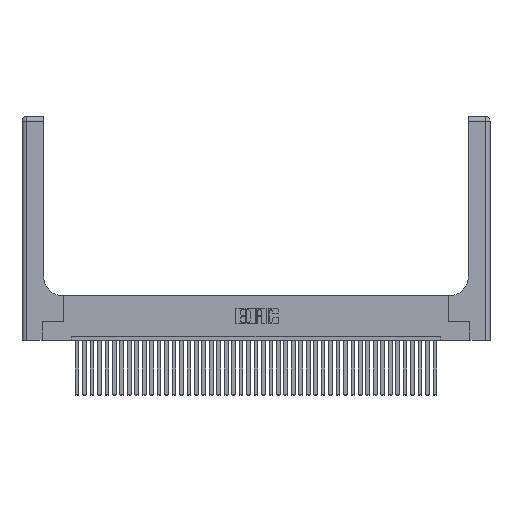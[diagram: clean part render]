
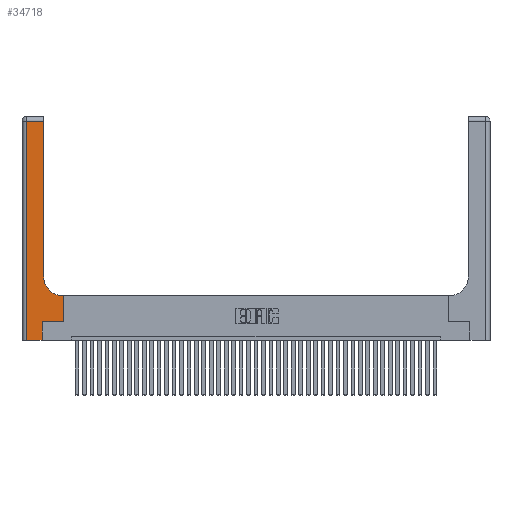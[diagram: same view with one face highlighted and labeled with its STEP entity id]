
A CAD part, top view. The second image highlights one B-rep face of the part: STEP entity #34718.
In plain terms, the highlighted planar face has unit normal (0, 0, 1).
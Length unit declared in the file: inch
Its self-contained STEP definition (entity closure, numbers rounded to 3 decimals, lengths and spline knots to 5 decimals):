
#1272 = CARTESIAN_POINT ( 'NONE',  ( 0.2915, 0.6, 0.37 ) ) ;
#2655 = VERTEX_POINT ( 'NONE', #16847 ) ;
#3575 = LINE ( 'NONE', #16869, #28385 ) ;
#3771 = ORIENTED_EDGE ( 'NONE', *, *, #38435, .T. ) ;
#3933 = CARTESIAN_POINT ( 'NONE',  ( 0.269, 0., 0.37 ) ) ;
#4809 = EDGE_CURVE ( 'NONE', #7875, #30289, #5449, .T. ) ;
#5449 = LINE ( 'NONE', #14029, #14894 ) ;
#6465 = VERTEX_POINT ( 'NONE', #39701 ) ;
#6599 = LINE ( 'NONE', #19191, #39219 ) ;
#6974 = DIRECTION ( 'NONE',  ( 0., 1., 0. ) ) ;
#7875 = VERTEX_POINT ( 'NONE', #32581 ) ;
#8042 = DIRECTION ( 'NONE',  ( 0., -1., 0. ) ) ;
#9629 = DIRECTION ( 'NONE',  ( 1., 0., 0. ) ) ;
#10398 = VERTEX_POINT ( 'NONE', #20556 ) ;
#10690 = DIRECTION ( 'NONE',  ( 0., 0., -1. ) ) ;
#11286 = EDGE_CURVE ( 'NONE', #2655, #16186, #33464, .T. ) ;
#11590 = ORIENTED_EDGE ( 'NONE', *, *, #12431, .T. ) ;
#11736 = EDGE_CURVE ( 'NONE', #14462, #38582, #13588, .T. ) ;
#12431 = EDGE_CURVE ( 'NONE', #23843, #10398, #6599, .T. ) ;
#13115 = EDGE_CURVE ( 'NONE', #30289, #6465, #3575, .T. ) ;
#13588 = LINE ( 'NONE', #1272, #25993 ) ;
#14029 = CARTESIAN_POINT ( 'NONE',  ( 0.2915, 3., 0.37 ) ) ;
#14373 = CARTESIAN_POINT ( 'NONE',  ( 0., 0., 0.37 ) ) ;
#14462 = VERTEX_POINT ( 'NONE', #20486 ) ;
#14894 = VECTOR ( 'NONE', #17952, 39.37008 ) ;
#15228 = ORIENTED_EDGE ( 'NONE', *, *, #34565, .T. ) ;
#15544 = CARTESIAN_POINT ( 'NONE',  ( 0.2915, 2.94, 0.37 ) ) ;
#16186 = VERTEX_POINT ( 'NONE', #3933 ) ;
#16752 = DIRECTION ( 'NONE',  ( 1., 0., 0. ) ) ;
#16847 = CARTESIAN_POINT ( 'NONE',  ( 0.06, 0., 0.37 ) ) ;
#16869 = CARTESIAN_POINT ( 'NONE',  ( 0., 2.94, 0.37 ) ) ;
#17952 = DIRECTION ( 'NONE',  ( 0., 1., 0. ) ) ;
#18336 = LINE ( 'NONE', #27028, #24257 ) ;
#19191 = CARTESIAN_POINT ( 'NONE',  ( 0.269, 0.25, 0.37 ) ) ;
#19296 = VECTOR ( 'NONE', #20844, 39.37008 ) ;
#19597 = CARTESIAN_POINT ( 'NONE',  ( 0.269, 0., 0.37 ) ) ;
#20119 = CARTESIAN_POINT ( 'NONE',  ( 0., 3., 0.37 ) ) ;
#20256 = PLANE ( 'NONE',  #32956 ) ;
#20486 = CARTESIAN_POINT ( 'NONE',  ( 0.5585, 0.6, 0.37 ) ) ;
#20556 = CARTESIAN_POINT ( 'NONE',  ( 0.5585, 0.25, 0.37 ) ) ;
#20844 = DIRECTION ( 'NONE',  ( 0., 1., 0. ) ) ;
#21967 = ORIENTED_EDGE ( 'NONE', *, *, #11736, .T. ) ;
#22255 = DIRECTION ( 'NONE',  ( 1., 0., 0. ) ) ;
#23441 = DIRECTION ( 'NONE',  ( -1., 0., 0. ) ) ;
#23508 = EDGE_LOOP ( 'NONE', ( #30646, #26108, #26517, #26839, #32368, #11590, #3771, #21967, #15228 ) ) ;
#23843 = VERTEX_POINT ( 'NONE', #37008 ) ;
#24257 = VECTOR ( 'NONE', #8042, 39.37008 ) ;
#25553 = EDGE_CURVE ( 'NONE', #6465, #2655, #18336, .T. ) ;
#25727 = CARTESIAN_POINT ( 'NONE',  ( 0.5415, 0.85, 0.37 ) ) ;
#25993 = VECTOR ( 'NONE', #37672, 39.37008 ) ;
#26108 = ORIENTED_EDGE ( 'NONE', *, *, #13115, .T. ) ;
#26517 = ORIENTED_EDGE ( 'NONE', *, *, #25553, .T. ) ;
#26839 = ORIENTED_EDGE ( 'NONE', *, *, #11286, .T. ) ;
#27028 = CARTESIAN_POINT ( 'NONE',  ( 0.06, 3., 0.37 ) ) ;
#27769 = LINE ( 'NONE', #39612, #19296 ) ;
#28385 = VECTOR ( 'NONE', #33182, 39.37008 ) ;
#30289 = VERTEX_POINT ( 'NONE', #15544 ) ;
#30646 = ORIENTED_EDGE ( 'NONE', *, *, #4809, .T. ) ;
#30971 = VECTOR ( 'NONE', #16752, 39.37008 ) ;
#31089 = CARTESIAN_POINT ( 'NONE',  ( 0.5415, 0.6, 0.37 ) ) ;
#32049 = DIRECTION ( 'NONE',  ( 0., 0., -1. ) ) ;
#32368 = ORIENTED_EDGE ( 'NONE', *, *, #40231, .T. ) ;
#32488 = LINE ( 'NONE', #19597, #36970 ) ;
#32581 = CARTESIAN_POINT ( 'NONE',  ( 0.2915, 0.85, 0.37 ) ) ;
#32956 = AXIS2_PLACEMENT_3D ( 'NONE', #20119, #10690, #23441 ) ;
#33182 = DIRECTION ( 'NONE',  ( -1., 0., 0. ) ) ;
#33457 = FACE_OUTER_BOUND ( 'NONE', #23508, .T. ) ;
#33464 = LINE ( 'NONE', #14373, #30971 ) ;
#34565 = EDGE_CURVE ( 'NONE', #38582, #7875, #40397, .T. ) ;
#34718 = ADVANCED_FACE ( 'NONE', ( #33457 ), #20256, .F. ) ;
#36385 = AXIS2_PLACEMENT_3D ( 'NONE', #25727, #32049, #22255 ) ;
#36970 = VECTOR ( 'NONE', #6974, 39.37008 ) ;
#37008 = CARTESIAN_POINT ( 'NONE',  ( 0.269, 0.25, 0.37 ) ) ;
#37672 = DIRECTION ( 'NONE',  ( -1., 0., 0. ) ) ;
#38435 = EDGE_CURVE ( 'NONE', #10398, #14462, #27769, .T. ) ;
#38582 = VERTEX_POINT ( 'NONE', #31089 ) ;
#39219 = VECTOR ( 'NONE', #9629, 39.37008 ) ;
#39612 = CARTESIAN_POINT ( 'NONE',  ( 0.5585, 0.25, 0.37 ) ) ;
#39701 = CARTESIAN_POINT ( 'NONE',  ( 0.06, 2.94, 0.37 ) ) ;
#40231 = EDGE_CURVE ( 'NONE', #16186, #23843, #32488, .T. ) ;
#40397 = CIRCLE ( 'NONE', #36385, 0.25 ) ;
